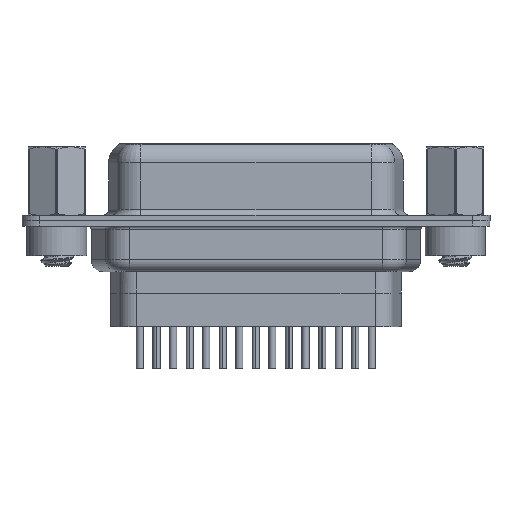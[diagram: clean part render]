
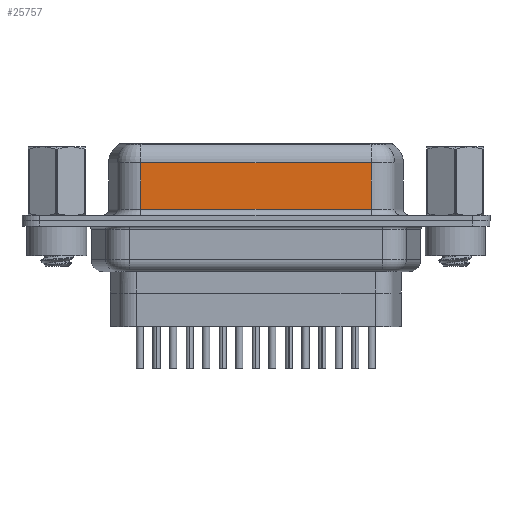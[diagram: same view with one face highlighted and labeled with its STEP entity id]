
A CAD part, front view. The second image highlights one B-rep face of the part: STEP entity #25757.
In plain terms, the highlighted planar face has unit normal (0, -1, 0).
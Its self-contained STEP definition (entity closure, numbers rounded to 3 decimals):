
#147 = CARTESIAN_POINT ( 'NONE',  ( 26.297, -3.95, 6.6 ) ) ;
#515 = CARTESIAN_POINT ( 'NONE',  ( 26.297, -3.95, 6.6 ) ) ;
#876 = CARTESIAN_POINT ( 'NONE',  ( 26.297, -3.95, 0.95 ) ) ;
#1164 = CARTESIAN_POINT ( 'NONE',  ( 7.023, -3.95, 0.95 ) ) ;
#1518 = EDGE_CURVE ( 'NONE', #21873, #27518, #21270, .T. ) ;
#1753 = ORIENTED_EDGE ( 'NONE', *, *, #12881, .T. ) ;
#2534 = VECTOR ( 'NONE', #9909, 1000. ) ;
#3604 = AXIS2_PLACEMENT_3D ( 'NONE', #147, #27844, #16216 ) ;
#8900 = DIRECTION ( 'NONE',  ( 0., 0., -1. ) ) ;
#8934 = FACE_OUTER_BOUND ( 'NONE', #17096, .T. ) ;
#8954 = CARTESIAN_POINT ( 'NONE',  ( 7.023, -3.95, 4.85 ) ) ;
#9211 = EDGE_CURVE ( 'NONE', #20808, #25093, #27510, .T. ) ;
#9909 = DIRECTION ( 'NONE',  ( 0., 0., -1. ) ) ;
#11994 = CARTESIAN_POINT ( 'NONE',  ( 26.297, -3.95, 0.95 ) ) ;
#12336 = ORIENTED_EDGE ( 'NONE', *, *, #1518, .F. ) ;
#12881 = EDGE_CURVE ( 'NONE', #21873, #20808, #20750, .T. ) ;
#14267 = LINE ( 'NONE', #11994, #19981 ) ;
#15655 = ORIENTED_EDGE ( 'NONE', *, *, #16608, .T. ) ;
#16216 = DIRECTION ( 'NONE',  ( 0., 0., 1. ) ) ;
#16608 = EDGE_CURVE ( 'NONE', #25093, #27518, #14267, .T. ) ;
#17096 = EDGE_LOOP ( 'NONE', ( #12336, #1753, #29757, #15655 ) ) ;
#19981 = VECTOR ( 'NONE', #23206, 1000. ) ;
#20750 = LINE ( 'NONE', #21195, #21760 ) ;
#20808 = VERTEX_POINT ( 'NONE', #8954 ) ;
#21195 = CARTESIAN_POINT ( 'NONE',  ( 26.297, -3.95, 4.85 ) ) ;
#21270 = LINE ( 'NONE', #515, #2534 ) ;
#21760 = VECTOR ( 'NONE', #23165, 1000. ) ;
#21873 = VERTEX_POINT ( 'NONE', #28604 ) ;
#22544 = CARTESIAN_POINT ( 'NONE',  ( 7.023, -3.95, 6.6 ) ) ;
#23165 = DIRECTION ( 'NONE',  ( -1., 0., 0. ) ) ;
#23206 = DIRECTION ( 'NONE',  ( 1., 0., 0. ) ) ;
#25093 = VERTEX_POINT ( 'NONE', #1164 ) ;
#25514 = VECTOR ( 'NONE', #8900, 1000. ) ;
#25573 = PLANE ( 'NONE',  #3604 ) ;
#25757 = ADVANCED_FACE ( 'NONE', ( #8934 ), #25573, .F. ) ;
#27510 = LINE ( 'NONE', #22544, #25514 ) ;
#27518 = VERTEX_POINT ( 'NONE', #876 ) ;
#27844 = DIRECTION ( 'NONE',  ( 0., 1., 0. ) ) ;
#28604 = CARTESIAN_POINT ( 'NONE',  ( 26.297, -3.95, 4.85 ) ) ;
#29757 = ORIENTED_EDGE ( 'NONE', *, *, #9211, .T. ) ;
